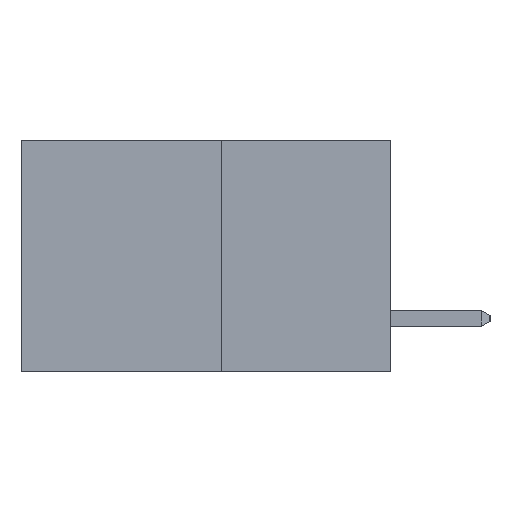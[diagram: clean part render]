
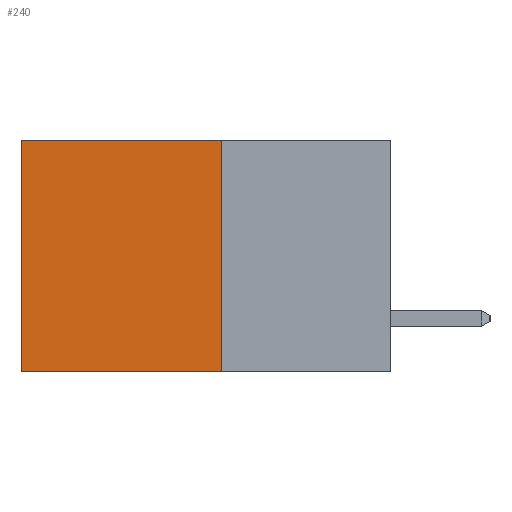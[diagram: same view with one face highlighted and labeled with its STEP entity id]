
A CAD part, left-side view. The second image highlights one B-rep face of the part: STEP entity #240.
In plain terms, the highlighted planar face has unit normal (-1, 0, 0).
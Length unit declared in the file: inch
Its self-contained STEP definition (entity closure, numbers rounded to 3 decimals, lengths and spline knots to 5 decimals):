
#188 = VERTEX_POINT ( 'NONE', #3409 ) ;
#240 = ADVANCED_FACE ( 'NONE', ( #1143 ), #5704, .F. ) ;
#919 = ORIENTED_EDGE ( 'NONE', *, *, #2934, .F. ) ;
#1143 = FACE_OUTER_BOUND ( 'NONE', #9347, .T. ) ;
#1248 = CARTESIAN_POINT ( 'NONE',  ( 0.277, 0.27, -0.37 ) ) ;
#1277 = CARTESIAN_POINT ( 'NONE',  ( 0.277, 0.27, -0.37 ) ) ;
#1574 = LINE ( 'NONE', #1248, #9875 ) ;
#1998 = VECTOR ( 'NONE', #7581, 39.37008 ) ;
#2145 = DIRECTION ( 'NONE',  ( 0., 1., 0. ) ) ;
#2160 = CARTESIAN_POINT ( 'NONE',  ( 0.277, 0.27, -0.37 ) ) ;
#2329 = LINE ( 'NONE', #7855, #6547 ) ;
#2560 = DIRECTION ( 'NONE',  ( 0., 1., 0. ) ) ;
#2934 = EDGE_CURVE ( 'NONE', #9312, #3501, #2329, .T. ) ;
#3248 = ORIENTED_EDGE ( 'NONE', *, *, #8597, .T. ) ;
#3409 = CARTESIAN_POINT ( 'NONE',  ( 0.277, 0.59, -0.37 ) ) ;
#3501 = VERTEX_POINT ( 'NONE', #1277 ) ;
#4649 = AXIS2_PLACEMENT_3D ( 'NONE', #2160, #5021, #5061 ) ;
#4991 = LINE ( 'NONE', #10773, #6928 ) ;
#5021 = DIRECTION ( 'NONE',  ( 1., 0., 0. ) ) ;
#5061 = DIRECTION ( 'NONE',  ( 0., 0., -1. ) ) ;
#5240 = ORIENTED_EDGE ( 'NONE', *, *, #9554, .F. ) ;
#5267 = EDGE_CURVE ( 'NONE', #8024, #188, #10819, .T. ) ;
#5704 = PLANE ( 'NONE',  #4649 ) ;
#6065 = CARTESIAN_POINT ( 'NONE',  ( 0.277, 0.27, 0. ) ) ;
#6547 = VECTOR ( 'NONE', #7778, 39.37008 ) ;
#6759 = CARTESIAN_POINT ( 'NONE',  ( 0.277, 0.59, -0.37 ) ) ;
#6928 = VECTOR ( 'NONE', #2560, 39.37008 ) ;
#7160 = ORIENTED_EDGE ( 'NONE', *, *, #5267, .T. ) ;
#7581 = DIRECTION ( 'NONE',  ( 0., 0., -1. ) ) ;
#7778 = DIRECTION ( 'NONE',  ( 0., 0., -1. ) ) ;
#7855 = CARTESIAN_POINT ( 'NONE',  ( 0.277, 0.27, -0.37 ) ) ;
#8024 = VERTEX_POINT ( 'NONE', #9231 ) ;
#8597 = EDGE_CURVE ( 'NONE', #9312, #8024, #4991, .T. ) ;
#9231 = CARTESIAN_POINT ( 'NONE',  ( 0.277, 0.59, 0. ) ) ;
#9312 = VERTEX_POINT ( 'NONE', #6065 ) ;
#9347 = EDGE_LOOP ( 'NONE', ( #7160, #5240, #919, #3248 ) ) ;
#9554 = EDGE_CURVE ( 'NONE', #3501, #188, #1574, .T. ) ;
#9875 = VECTOR ( 'NONE', #2145, 39.37008 ) ;
#10773 = CARTESIAN_POINT ( 'NONE',  ( 0.277, 0.27, 0. ) ) ;
#10819 = LINE ( 'NONE', #6759, #1998 ) ;
